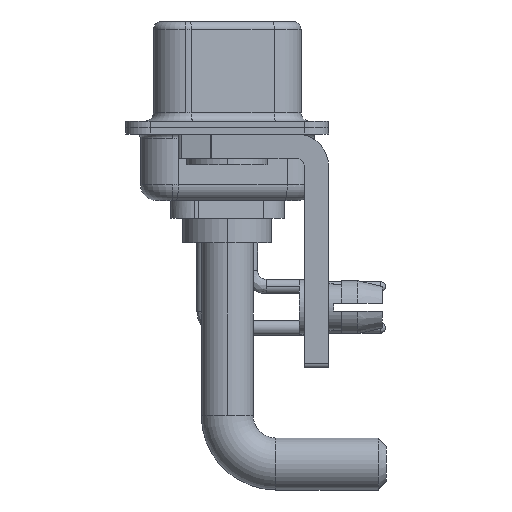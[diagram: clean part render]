
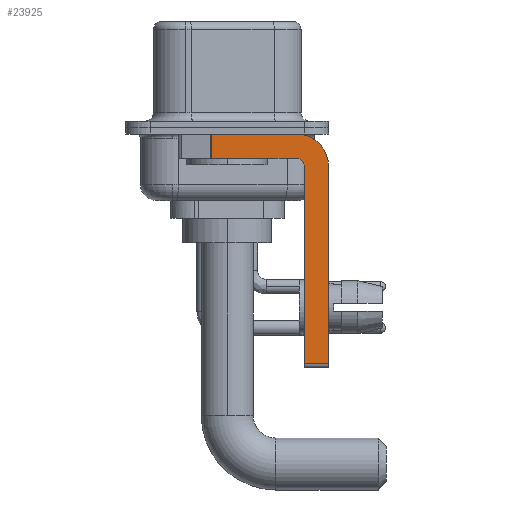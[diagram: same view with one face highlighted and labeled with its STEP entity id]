
A CAD part, left-side view. The second image highlights one B-rep face of the part: STEP entity #23925.
In plain terms, the highlighted planar face has unit normal (-1, 0, 0).
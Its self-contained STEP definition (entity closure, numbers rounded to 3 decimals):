
#64 = PLANE ( 'NONE',  #9646 ) ;
#1235 = CARTESIAN_POINT ( 'NONE',  ( -2.9, -6.25, -2.4 ) ) ;
#1317 = EDGE_CURVE ( 'NONE', #20436, #13101, #23750, .T. ) ;
#1434 = EDGE_CURVE ( 'NONE', #14461, #12356, #19880, .T. ) ;
#1448 = CARTESIAN_POINT ( 'NONE',  ( -2.9, -4.25, -2.4 ) ) ;
#2398 = VERTEX_POINT ( 'NONE', #5058 ) ;
#2442 = VECTOR ( 'NONE', #15761, 1000. ) ;
#2550 = LINE ( 'NONE', #4851, #15750 ) ;
#2680 = CARTESIAN_POINT ( 'NONE',  ( -2.9, -4.25, -0.4 ) ) ;
#3423 = CARTESIAN_POINT ( 'NONE',  ( -2.9, -4.25, -1.9 ) ) ;
#4214 = LINE ( 'NONE', #25014, #19843 ) ;
#4721 = DIRECTION ( 'NONE',  ( 0., 0., -1. ) ) ;
#4851 = CARTESIAN_POINT ( 'NONE',  ( -2.9, -6.25, -2.4 ) ) ;
#5058 = CARTESIAN_POINT ( 'NONE',  ( -2.9, 0.978, -1.9 ) ) ;
#5557 = DIRECTION ( 'NONE',  ( 0., 0., -1. ) ) ;
#5668 = DIRECTION ( 'NONE',  ( 0., 0., -1. ) ) ;
#5800 = CIRCLE ( 'NONE', #23158, 0.5 ) ;
#5909 = ORIENTED_EDGE ( 'NONE', *, *, #12544, .F. ) ;
#6376 = DIRECTION ( 'NONE',  ( 0., -1., 0. ) ) ;
#6471 = VERTEX_POINT ( 'NONE', #3423 ) ;
#6836 = AXIS2_PLACEMENT_3D ( 'NONE', #24298, #8259, #5668 ) ;
#8259 = DIRECTION ( 'NONE',  ( 1., 0., 0. ) ) ;
#8360 = DIRECTION ( 'NONE',  ( 1., 0., 0. ) ) ;
#9314 = EDGE_CURVE ( 'NONE', #16501, #2398, #26348, .T. ) ;
#9646 = AXIS2_PLACEMENT_3D ( 'NONE', #18426, #8360, #16675 ) ;
#9726 = DIRECTION ( 'NONE',  ( -1., 0., 0. ) ) ;
#10939 = VERTEX_POINT ( 'NONE', #14957 ) ;
#11475 = EDGE_LOOP ( 'NONE', ( #5909, #20321, #19867, #21065, #22282, #21151, #14862, #12890 ) ) ;
#11493 = EDGE_CURVE ( 'NONE', #6471, #2398, #17912, .T. ) ;
#12356 = VERTEX_POINT ( 'NONE', #1235 ) ;
#12544 = EDGE_CURVE ( 'NONE', #16501, #14461, #4214, .T. ) ;
#12616 = CARTESIAN_POINT ( 'NONE',  ( -2.9, -4.75, -2.4 ) ) ;
#12890 = ORIENTED_EDGE ( 'NONE', *, *, #1434, .F. ) ;
#13101 = VERTEX_POINT ( 'NONE', #12616 ) ;
#14461 = VERTEX_POINT ( 'NONE', #2680 ) ;
#14844 = CARTESIAN_POINT ( 'NONE',  ( -2.9, -4.75, -14.55 ) ) ;
#14862 = ORIENTED_EDGE ( 'NONE', *, *, #19278, .F. ) ;
#14906 = FACE_OUTER_BOUND ( 'NONE', #11475, .T. ) ;
#14957 = CARTESIAN_POINT ( 'NONE',  ( -2.9, -6.25, -14.55 ) ) ;
#15561 = VECTOR ( 'NONE', #25668, 1000. ) ;
#15750 = VECTOR ( 'NONE', #4721, 1000. ) ;
#15761 = DIRECTION ( 'NONE',  ( 0., 1., 0. ) ) ;
#16501 = VERTEX_POINT ( 'NONE', #21217 ) ;
#16675 = DIRECTION ( 'NONE',  ( 0., 0., -1. ) ) ;
#17912 = LINE ( 'NONE', #20220, #2442 ) ;
#18162 = DIRECTION ( 'NONE',  ( 0., 0., 1. ) ) ;
#18426 = CARTESIAN_POINT ( 'NONE',  ( -2.9, -4.25, -2.4 ) ) ;
#19278 = EDGE_CURVE ( 'NONE', #12356, #10939, #2550, .T. ) ;
#19432 = DIRECTION ( 'NONE',  ( 0., -1., 0. ) ) ;
#19843 = VECTOR ( 'NONE', #6376, 1000. ) ;
#19867 = ORIENTED_EDGE ( 'NONE', *, *, #11493, .F. ) ;
#19880 = CIRCLE ( 'NONE', #6836, 2. ) ;
#20220 = CARTESIAN_POINT ( 'NONE',  ( -2.9, -4.25, -1.9 ) ) ;
#20321 = ORIENTED_EDGE ( 'NONE', *, *, #9314, .T. ) ;
#20436 = VERTEX_POINT ( 'NONE', #14844 ) ;
#21065 = ORIENTED_EDGE ( 'NONE', *, *, #21907, .F. ) ;
#21151 = ORIENTED_EDGE ( 'NONE', *, *, #26248, .T. ) ;
#21217 = CARTESIAN_POINT ( 'NONE',  ( -2.9, 0.978, -0.4 ) ) ;
#21842 = CARTESIAN_POINT ( 'NONE',  ( -2.9, -4.75, -14.8 ) ) ;
#21907 = EDGE_CURVE ( 'NONE', #13101, #6471, #5800, .T. ) ;
#22271 = VECTOR ( 'NONE', #19432, 1000. ) ;
#22282 = ORIENTED_EDGE ( 'NONE', *, *, #1317, .F. ) ;
#23158 = AXIS2_PLACEMENT_3D ( 'NONE', #1448, #9726, #18162 ) ;
#23236 = CARTESIAN_POINT ( 'NONE',  ( -2.9, -4.25, -14.55 ) ) ;
#23750 = LINE ( 'NONE', #21842, #15561 ) ;
#23925 = ADVANCED_FACE ( 'NONE', ( #14906 ), #64, .F. ) ;
#24298 = CARTESIAN_POINT ( 'NONE',  ( -2.9, -4.25, -2.4 ) ) ;
#25014 = CARTESIAN_POINT ( 'NONE',  ( -2.9, 3., -0.4 ) ) ;
#25396 = VECTOR ( 'NONE', #5557, 1000. ) ;
#25546 = LINE ( 'NONE', #23236, #22271 ) ;
#25668 = DIRECTION ( 'NONE',  ( 0., 0., 1. ) ) ;
#26075 = CARTESIAN_POINT ( 'NONE',  ( -2.9, 0.978, -1.9 ) ) ;
#26248 = EDGE_CURVE ( 'NONE', #20436, #10939, #25546, .T. ) ;
#26348 = LINE ( 'NONE', #26075, #25396 ) ;
